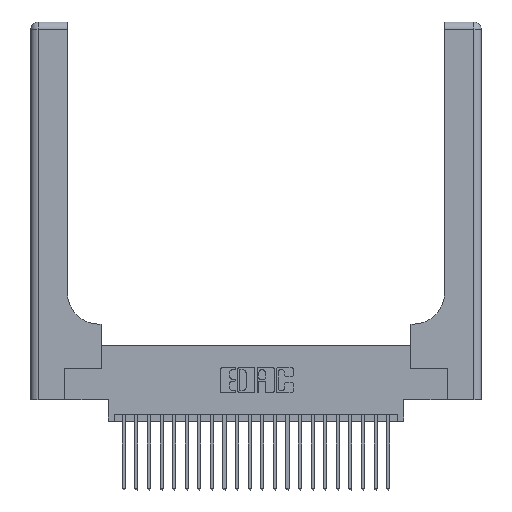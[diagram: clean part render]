
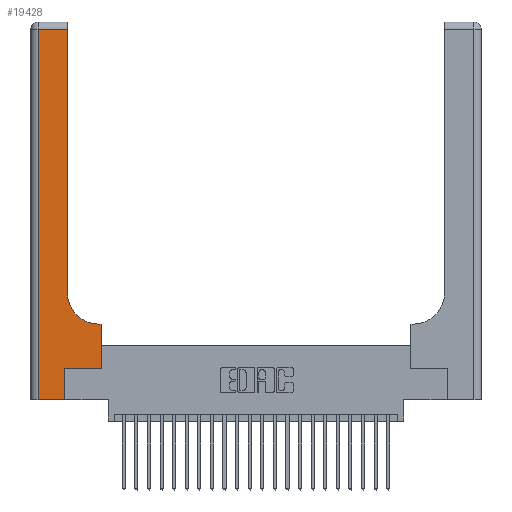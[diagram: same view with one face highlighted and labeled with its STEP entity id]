
A CAD part, top view. The second image highlights one B-rep face of the part: STEP entity #19428.
In plain terms, the highlighted planar face has unit normal (0, 0, 1).
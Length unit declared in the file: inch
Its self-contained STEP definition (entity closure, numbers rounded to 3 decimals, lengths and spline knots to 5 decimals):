
#58 = VECTOR ( 'NONE', #5259, 39.37008 ) ;
#90 = DIRECTION ( 'NONE',  ( 1., 0., 0. ) ) ;
#141 = EDGE_CURVE ( 'NONE', #772, #20299, #10047, .T. ) ;
#400 = ORIENTED_EDGE ( 'NONE', *, *, #12784, .T. ) ;
#631 = CARTESIAN_POINT ( 'NONE',  ( 0.5585, 0.6, 0.37 ) ) ;
#671 = LINE ( 'NONE', #14851, #58 ) ;
#772 = VERTEX_POINT ( 'NONE', #12791 ) ;
#824 = VERTEX_POINT ( 'NONE', #25053 ) ;
#1510 = VECTOR ( 'NONE', #24064, 39.37008 ) ;
#1902 = DIRECTION ( 'NONE',  ( -1., 0., 0. ) ) ;
#2298 = LINE ( 'NONE', #4092, #16068 ) ;
#2494 = DIRECTION ( 'NONE',  ( -1., 0., 0. ) ) ;
#3111 = VERTEX_POINT ( 'NONE', #3462 ) ;
#3462 = CARTESIAN_POINT ( 'NONE',  ( 0.2915, 0.85, 0.37 ) ) ;
#4092 = CARTESIAN_POINT ( 'NONE',  ( 0.2915, 0.6, 0.37 ) ) ;
#4230 = EDGE_CURVE ( 'NONE', #824, #3111, #18444, .T. ) ;
#4293 = DIRECTION ( 'NONE',  ( 1., 0., 0. ) ) ;
#4419 = ORIENTED_EDGE ( 'NONE', *, *, #19236, .T. ) ;
#4721 = PLANE ( 'NONE',  #19740 ) ;
#5259 = DIRECTION ( 'NONE',  ( 1., 0., 0. ) ) ;
#5354 = VERTEX_POINT ( 'NONE', #21076 ) ;
#5796 = DIRECTION ( 'NONE',  ( -1., 0., 0. ) ) ;
#5955 = ORIENTED_EDGE ( 'NONE', *, *, #24404, .T. ) ;
#6175 = CARTESIAN_POINT ( 'NONE',  ( 0.5415, 0.85, 0.37 ) ) ;
#6666 = DIRECTION ( 'NONE',  ( 0., 0., -1. ) ) ;
#7495 = VECTOR ( 'NONE', #1902, 39.37008 ) ;
#8620 = ORIENTED_EDGE ( 'NONE', *, *, #141, .T. ) ;
#8674 = VERTEX_POINT ( 'NONE', #23910 ) ;
#9028 = VERTEX_POINT ( 'NONE', #23129 ) ;
#9460 = AXIS2_PLACEMENT_3D ( 'NONE', #6175, #13875, #4293 ) ;
#10047 = LINE ( 'NONE', #21872, #1510 ) ;
#10132 = VECTOR ( 'NONE', #15894, 39.37008 ) ;
#10824 = CARTESIAN_POINT ( 'NONE',  ( 0.2915, 3., 0.37 ) ) ;
#11462 = VECTOR ( 'NONE', #22198, 39.37008 ) ;
#11759 = CARTESIAN_POINT ( 'NONE',  ( 0., 0., 0.37 ) ) ;
#11832 = CARTESIAN_POINT ( 'NONE',  ( 0.5585, 0.25, 0.37 ) ) ;
#12303 = CARTESIAN_POINT ( 'NONE',  ( 0., 3., 0.37 ) ) ;
#12648 = VECTOR ( 'NONE', #90, 39.37008 ) ;
#12657 = FACE_OUTER_BOUND ( 'NONE', #17169, .T. ) ;
#12784 = EDGE_CURVE ( 'NONE', #20299, #9028, #671, .T. ) ;
#12791 = CARTESIAN_POINT ( 'NONE',  ( 0.269, 0., 0.37 ) ) ;
#12945 = LINE ( 'NONE', #11759, #12648 ) ;
#13015 = LINE ( 'NONE', #10824, #15171 ) ;
#13611 = CARTESIAN_POINT ( 'NONE',  ( 0., 2.94, 0.37 ) ) ;
#13852 = ORIENTED_EDGE ( 'NONE', *, *, #19838, .T. ) ;
#13875 = DIRECTION ( 'NONE',  ( 0., 0., -1. ) ) ;
#14851 = CARTESIAN_POINT ( 'NONE',  ( 0.269, 0.25, 0.37 ) ) ;
#15171 = VECTOR ( 'NONE', #24431, 39.37008 ) ;
#15894 = DIRECTION ( 'NONE',  ( 0., 1., 0. ) ) ;
#15987 = ORIENTED_EDGE ( 'NONE', *, *, #23299, .T. ) ;
#16068 = VECTOR ( 'NONE', #5796, 39.37008 ) ;
#16401 = LINE ( 'NONE', #13611, #7495 ) ;
#17169 = EDGE_LOOP ( 'NONE', ( #15987, #4419, #17326, #5955, #8620, #400, #23281, #13852, #18388 ) ) ;
#17326 = ORIENTED_EDGE ( 'NONE', *, *, #18754, .T. ) ;
#18259 = VERTEX_POINT ( 'NONE', #23833 ) ;
#18388 = ORIENTED_EDGE ( 'NONE', *, *, #4230, .T. ) ;
#18444 = CIRCLE ( 'NONE', #9460, 0.25 ) ;
#18754 = EDGE_CURVE ( 'NONE', #8674, #5354, #25253, .T. ) ;
#19236 = EDGE_CURVE ( 'NONE', #18259, #8674, #16401, .T. ) ;
#19428 = ADVANCED_FACE ( 'NONE', ( #12657 ), #4721, .F. ) ;
#19445 = VERTEX_POINT ( 'NONE', #631 ) ;
#19740 = AXIS2_PLACEMENT_3D ( 'NONE', #12303, #6666, #2494 ) ;
#19838 = EDGE_CURVE ( 'NONE', #19445, #824, #2298, .T. ) ;
#20299 = VERTEX_POINT ( 'NONE', #21224 ) ;
#21076 = CARTESIAN_POINT ( 'NONE',  ( 0.06, 0., 0.37 ) ) ;
#21224 = CARTESIAN_POINT ( 'NONE',  ( 0.269, 0.25, 0.37 ) ) ;
#21872 = CARTESIAN_POINT ( 'NONE',  ( 0.269, 0., 0.37 ) ) ;
#21897 = EDGE_CURVE ( 'NONE', #9028, #19445, #23917, .T. ) ;
#22198 = DIRECTION ( 'NONE',  ( 0., -1., 0. ) ) ;
#23129 = CARTESIAN_POINT ( 'NONE',  ( 0.5585, 0.25, 0.37 ) ) ;
#23281 = ORIENTED_EDGE ( 'NONE', *, *, #21897, .T. ) ;
#23299 = EDGE_CURVE ( 'NONE', #3111, #18259, #13015, .T. ) ;
#23833 = CARTESIAN_POINT ( 'NONE',  ( 0.2915, 2.94, 0.37 ) ) ;
#23910 = CARTESIAN_POINT ( 'NONE',  ( 0.06, 2.94, 0.37 ) ) ;
#23917 = LINE ( 'NONE', #11832, #10132 ) ;
#24064 = DIRECTION ( 'NONE',  ( 0., 1., 0. ) ) ;
#24142 = CARTESIAN_POINT ( 'NONE',  ( 0.06, 3., 0.37 ) ) ;
#24404 = EDGE_CURVE ( 'NONE', #5354, #772, #12945, .T. ) ;
#24431 = DIRECTION ( 'NONE',  ( 0., 1., 0. ) ) ;
#25053 = CARTESIAN_POINT ( 'NONE',  ( 0.5415, 0.6, 0.37 ) ) ;
#25253 = LINE ( 'NONE', #24142, #11462 ) ;
